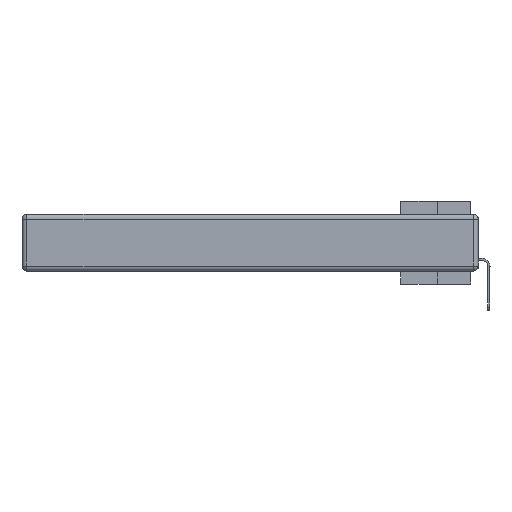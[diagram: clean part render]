
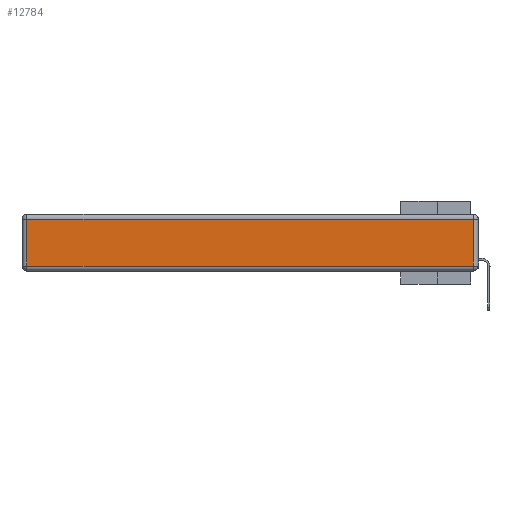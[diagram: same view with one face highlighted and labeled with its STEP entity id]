
A CAD part, left-side view. The second image highlights one B-rep face of the part: STEP entity #12784.
In plain terms, the highlighted planar face has unit normal (-1, 0, 0).
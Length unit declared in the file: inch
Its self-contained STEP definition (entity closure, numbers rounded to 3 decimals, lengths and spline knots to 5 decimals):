
#400 = DIRECTION ( 'NONE',  ( 0., 0., -1. ) ) ;
#1827 = LINE ( 'NONE', #14441, #23972 ) ;
#2869 = LINE ( 'NONE', #9553, #11154 ) ;
#2901 = VERTEX_POINT ( 'NONE', #8834 ) ;
#3298 = VERTEX_POINT ( 'NONE', #24692 ) ;
#5038 = LINE ( 'NONE', #13447, #25482 ) ;
#6588 = EDGE_CURVE ( 'NONE', #2901, #12166, #5038, .T. ) ;
#6641 = CARTESIAN_POINT ( 'NONE',  ( 0., 0.03, -0.313 ) ) ;
#8406 = ORIENTED_EDGE ( 'NONE', *, *, #19797, .T. ) ;
#8834 = CARTESIAN_POINT ( 'NONE',  ( 0., 2.72, -0.03 ) ) ;
#9148 = FACE_OUTER_BOUND ( 'NONE', #10929, .T. ) ;
#9553 = CARTESIAN_POINT ( 'NONE',  ( 0., 2.75, -0.03 ) ) ;
#10929 = EDGE_LOOP ( 'NONE', ( #13376, #13470, #8406, #16914 ) ) ;
#11154 = VECTOR ( 'NONE', #15615, 39.37008 ) ;
#11468 = DIRECTION ( 'NONE',  ( 0., 0., 1. ) ) ;
#12166 = VERTEX_POINT ( 'NONE', #20018 ) ;
#12761 = VECTOR ( 'NONE', #16669, 39.37008 ) ;
#12784 = ADVANCED_FACE ( 'NONE', ( #9148 ), #27377, .T. ) ;
#13376 = ORIENTED_EDGE ( 'NONE', *, *, #17930, .T. ) ;
#13447 = CARTESIAN_POINT ( 'NONE',  ( 0., 2.72, -0.343 ) ) ;
#13470 = ORIENTED_EDGE ( 'NONE', *, *, #14180, .T. ) ;
#13768 = CARTESIAN_POINT ( 'NONE',  ( 0., 0., -0.343 ) ) ;
#14180 = EDGE_CURVE ( 'NONE', #27655, #3298, #28085, .T. ) ;
#14441 = CARTESIAN_POINT ( 'NONE',  ( 0., 0., -0.313 ) ) ;
#15615 = DIRECTION ( 'NONE',  ( 0., 1., 0. ) ) ;
#16669 = DIRECTION ( 'NONE',  ( 0., 0., 1. ) ) ;
#16914 = ORIENTED_EDGE ( 'NONE', *, *, #6588, .T. ) ;
#17175 = DIRECTION ( 'NONE',  ( 0., -1., 0. ) ) ;
#17930 = EDGE_CURVE ( 'NONE', #12166, #27655, #1827, .T. ) ;
#19797 = EDGE_CURVE ( 'NONE', #3298, #2901, #2869, .T. ) ;
#20018 = CARTESIAN_POINT ( 'NONE',  ( 0., 2.72, -0.313 ) ) ;
#21420 = CARTESIAN_POINT ( 'NONE',  ( 0., 0.03, -0.343 ) ) ;
#22438 = DIRECTION ( 'NONE',  ( -1., 0., 0. ) ) ;
#23972 = VECTOR ( 'NONE', #17175, 39.37008 ) ;
#24692 = CARTESIAN_POINT ( 'NONE',  ( 0., 0.03, -0.03 ) ) ;
#25482 = VECTOR ( 'NONE', #400, 39.37008 ) ;
#25683 = AXIS2_PLACEMENT_3D ( 'NONE', #13768, #22438, #11468 ) ;
#27377 = PLANE ( 'NONE',  #25683 ) ;
#27655 = VERTEX_POINT ( 'NONE', #6641 ) ;
#28085 = LINE ( 'NONE', #21420, #12761 ) ;
